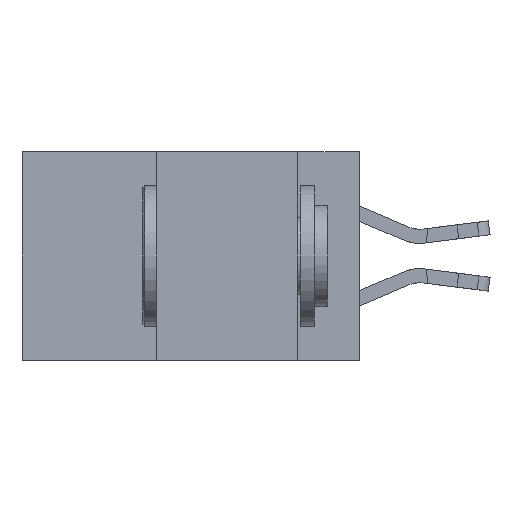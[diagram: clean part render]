
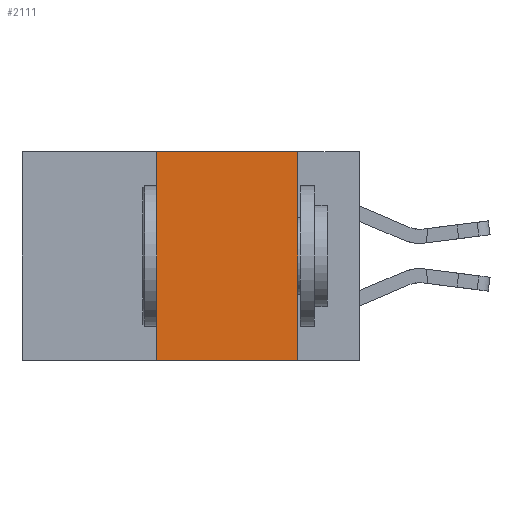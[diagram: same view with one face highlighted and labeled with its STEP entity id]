
A CAD part, left-side view. The second image highlights one B-rep face of the part: STEP entity #2111.
In plain terms, the highlighted planar face has unit normal (-1, 0, 0).
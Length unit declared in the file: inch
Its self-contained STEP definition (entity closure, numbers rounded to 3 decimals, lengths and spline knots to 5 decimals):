
#1164 = VERTEX_POINT ( 'NONE', #15366 ) ;
#1347 = LINE ( 'NONE', #15685, #10830 ) ;
#1510 = VERTEX_POINT ( 'NONE', #11775 ) ;
#1764 = DIRECTION ( 'NONE',  ( 0., 0., -1. ) ) ;
#2111 = ADVANCED_FACE ( 'NONE', ( #13273 ), #16282, .F. ) ;
#3523 = VECTOR ( 'NONE', #4691, 39.37008 ) ;
#3791 = EDGE_CURVE ( 'NONE', #1164, #13454, #6323, .T. ) ;
#3932 = LINE ( 'NONE', #12283, #3523 ) ;
#4013 = DIRECTION ( 'NONE',  ( 0., -1., 0. ) ) ;
#4691 = DIRECTION ( 'NONE',  ( 0., 0., 1. ) ) ;
#5133 = CARTESIAN_POINT ( 'NONE',  ( 0., 0.11, -0.37 ) ) ;
#5610 = DIRECTION ( 'NONE',  ( 0., -1., 0. ) ) ;
#6323 = LINE ( 'NONE', #9661, #16348 ) ;
#7298 = CARTESIAN_POINT ( 'NONE',  ( 0., 0.36, -0.37 ) ) ;
#7428 = AXIS2_PLACEMENT_3D ( 'NONE', #15509, #13586, #1764 ) ;
#7692 = EDGE_CURVE ( 'NONE', #15363, #13454, #16241, .T. ) ;
#7890 = CARTESIAN_POINT ( 'NONE',  ( 0., 0.6, -0.37 ) ) ;
#8403 = DIRECTION ( 'NONE',  ( 0., 0., -1. ) ) ;
#8775 = ORIENTED_EDGE ( 'NONE', *, *, #3791, .F. ) ;
#9080 = ORIENTED_EDGE ( 'NONE', *, *, #12367, .F. ) ;
#9149 = ORIENTED_EDGE ( 'NONE', *, *, #9207, .F. ) ;
#9162 = ORIENTED_EDGE ( 'NONE', *, *, #7692, .T. ) ;
#9207 = EDGE_CURVE ( 'NONE', #15363, #1510, #3932, .T. ) ;
#9661 = CARTESIAN_POINT ( 'NONE',  ( 0., 0.11, 0. ) ) ;
#10830 = VECTOR ( 'NONE', #5610, 39.37008 ) ;
#11775 = CARTESIAN_POINT ( 'NONE',  ( 0., 0.36, 0. ) ) ;
#12283 = CARTESIAN_POINT ( 'NONE',  ( 0., 0.36, 0. ) ) ;
#12367 = EDGE_CURVE ( 'NONE', #1510, #1164, #1347, .T. ) ;
#12906 = VECTOR ( 'NONE', #4013, 39.37008 ) ;
#13101 = EDGE_LOOP ( 'NONE', ( #8775, #9080, #9149, #9162 ) ) ;
#13273 = FACE_OUTER_BOUND ( 'NONE', #13101, .T. ) ;
#13454 = VERTEX_POINT ( 'NONE', #5133 ) ;
#13586 = DIRECTION ( 'NONE',  ( 1., 0., 0. ) ) ;
#15363 = VERTEX_POINT ( 'NONE', #7298 ) ;
#15366 = CARTESIAN_POINT ( 'NONE',  ( 0., 0.11, 0. ) ) ;
#15509 = CARTESIAN_POINT ( 'NONE',  ( 0., 0.6, 0. ) ) ;
#15685 = CARTESIAN_POINT ( 'NONE',  ( 0., 0.6, 0. ) ) ;
#16241 = LINE ( 'NONE', #7890, #12906 ) ;
#16282 = PLANE ( 'NONE',  #7428 ) ;
#16348 = VECTOR ( 'NONE', #8403, 39.37008 ) ;
